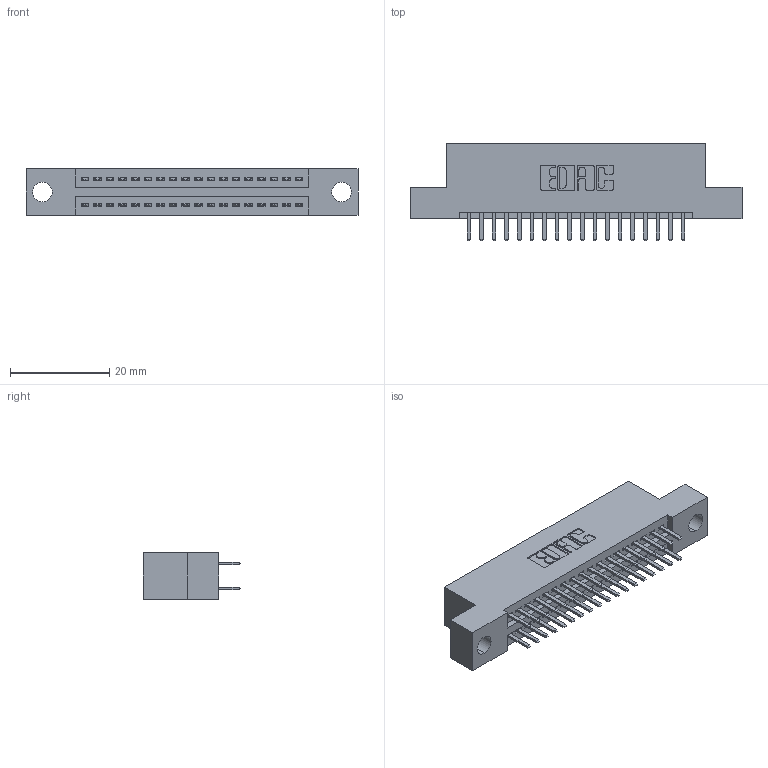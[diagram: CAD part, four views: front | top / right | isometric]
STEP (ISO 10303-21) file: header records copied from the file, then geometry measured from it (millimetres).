
FILE_DESCRIPTION (( 'STEP AP203' ), '1' );
FILE_NAME ('395-036-520-204.STEP', '2018-11-13T17:37:44', ( '' ), ( '' ), 'SwSTEP 2.0', 'SolidWorks 2016', '' );
FILE_SCHEMA (( 'CONFIG_CONTROL_DESIGN' ));
Length unit declared in the file: inch
Products named in the file (3): 345-292-001_345-293-120; 345 Part_Flush Mounting Lugs - 0.156 Dia-TH; 395-036-520-204
Assembly tree (37 placements, depth 2):
  395-036-520-204
    345 Part_Flush Mounting Lugs - 0.156 Dia-TH
    345-292-001_345-293-120  x36
Bounding box: 66.93 x 19.68 x 9.4 mm (x, y, z)
Volume: 6175.1 mm3; surface area: 8444.5 mm2
Topology: 37 solids, 37 shells, 2070 faces, 5993 edges, 3898 vertices
Faces by surface type: plane 1340, cylinder 730
Entity records: 17471 total; most frequent: CARTESIAN_POINT 2964, ORIENTED_EDGE 2886, DIRECTION 2631, EDGE_CURVE 1443, LINE 1235, VECTOR 1235, VERTEX_POINT 958, AXIS2_PLACEMENT_3D 698
